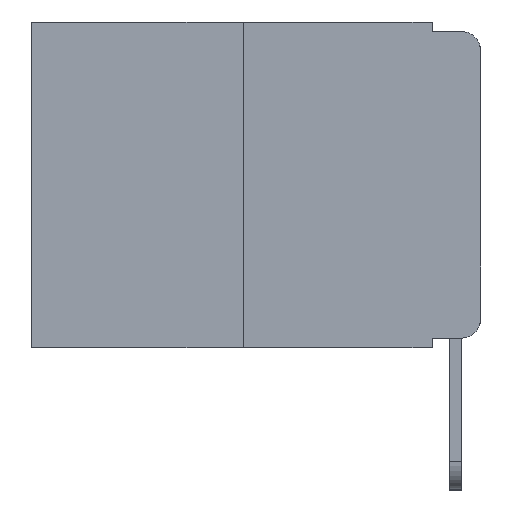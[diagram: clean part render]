
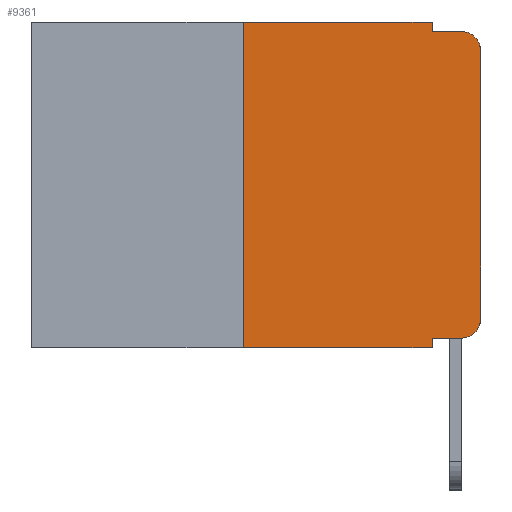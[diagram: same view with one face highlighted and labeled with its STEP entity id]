
A CAD part, left-side view. The second image highlights one B-rep face of the part: STEP entity #9361.
In plain terms, the highlighted planar face has unit normal (-1, 0, 0).
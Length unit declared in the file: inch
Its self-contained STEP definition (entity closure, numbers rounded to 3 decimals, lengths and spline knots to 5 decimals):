
#480 = LINE ( 'NONE', #10778, #15627 ) ;
#1045 = CARTESIAN_POINT ( 'NONE',  ( 0., 0.051, 0. ) ) ;
#1792 = CARTESIAN_POINT ( 'NONE',  ( 0., 0.051, -0.01 ) ) ;
#1855 = DIRECTION ( 'NONE',  ( 0., 0., -1. ) ) ;
#2043 = EDGE_CURVE ( 'NONE', #19481, #11397, #15780, .T. ) ;
#2341 = LINE ( 'NONE', #15578, #12651 ) ;
#2442 = LINE ( 'NONE', #15552, #7257 ) ;
#3213 = DIRECTION ( 'NONE',  ( 0., 0., -1. ) ) ;
#3222 = CARTESIAN_POINT ( 'NONE',  ( 0., 0.02, -0.333 ) ) ;
#4673 = ORIENTED_EDGE ( 'NONE', *, *, #9066, .F. ) ;
#4985 = ORIENTED_EDGE ( 'NONE', *, *, #9174, .F. ) ;
#5011 = ORIENTED_EDGE ( 'NONE', *, *, #9202, .F. ) ;
#5199 = CARTESIAN_POINT ( 'NONE',  ( 0., 0.25, 0. ) ) ;
#5466 = ORIENTED_EDGE ( 'NONE', *, *, #7893, .F. ) ;
#5467 = ORIENTED_EDGE ( 'NONE', *, *, #9296, .T. ) ;
#5751 = VERTEX_POINT ( 'NONE', #23654 ) ;
#5756 = CARTESIAN_POINT ( 'NONE',  ( 0., 0.02, -0.01 ) ) ;
#6042 = VERTEX_POINT ( 'NONE', #3222 ) ;
#6256 = DIRECTION ( 'NONE',  ( 0., 0., 1. ) ) ;
#6399 = ORIENTED_EDGE ( 'NONE', *, *, #9549, .T. ) ;
#6518 = CARTESIAN_POINT ( 'NONE',  ( 0., 0.051, -0.343 ) ) ;
#6658 = AXIS2_PLACEMENT_3D ( 'NONE', #19678, #8766, #21361 ) ;
#6812 = EDGE_CURVE ( 'NONE', #6042, #5751, #7649, .T. ) ;
#6962 = CARTESIAN_POINT ( 'NONE',  ( 0., 0.25, 0. ) ) ;
#7003 = EDGE_CURVE ( 'NONE', #19045, #6042, #480, .T. ) ;
#7114 = CARTESIAN_POINT ( 'NONE',  ( 0., 0.25, -0.343 ) ) ;
#7257 = VECTOR ( 'NONE', #1855, 39.37008 ) ;
#7326 = DIRECTION ( 'NONE',  ( 0., -1., 0. ) ) ;
#7649 = CIRCLE ( 'NONE', #11086, 0.02 ) ;
#7893 = EDGE_CURVE ( 'NONE', #19045, #11397, #2442, .T. ) ;
#8121 = VECTOR ( 'NONE', #3213, 39.37008 ) ;
#8412 = LINE ( 'NONE', #1792, #22184 ) ;
#8766 = DIRECTION ( 'NONE',  ( -1., 0., 0. ) ) ;
#9027 = EDGE_CURVE ( 'NONE', #19481, #18231, #9363, .T. ) ;
#9059 = CIRCLE ( 'NONE', #6658, 0.02 ) ;
#9066 = EDGE_CURVE ( 'NONE', #23045, #13034, #18016, .T. ) ;
#9174 = EDGE_CURVE ( 'NONE', #13034, #21559, #8412, .T. ) ;
#9202 = EDGE_CURVE ( 'NONE', #18231, #23045, #2341, .T. ) ;
#9242 = ORIENTED_EDGE ( 'NONE', *, *, #2043, .T. ) ;
#9296 = EDGE_CURVE ( 'NONE', #11720, #21559, #9059, .T. ) ;
#9361 = ADVANCED_FACE ( 'NONE', ( #20659 ), #16520, .F. ) ;
#9363 = LINE ( 'NONE', #5199, #19080 ) ;
#9549 = EDGE_CURVE ( 'NONE', #5751, #11720, #17179, .T. ) ;
#9937 = DIRECTION ( 'NONE',  ( 0., -1., 0. ) ) ;
#10778 = CARTESIAN_POINT ( 'NONE',  ( 0., 0.051, -0.333 ) ) ;
#10800 = ORIENTED_EDGE ( 'NONE', *, *, #9027, .F. ) ;
#10909 = DIRECTION ( 'NONE',  ( -1., 0., 0. ) ) ;
#11005 = DIRECTION ( 'NONE',  ( 1., 0., 0. ) ) ;
#11086 = AXIS2_PLACEMENT_3D ( 'NONE', #21469, #10909, #23155 ) ;
#11294 = CARTESIAN_POINT ( 'NONE',  ( 0., 0.473, -0.343 ) ) ;
#11397 = VERTEX_POINT ( 'NONE', #6518 ) ;
#11720 = VERTEX_POINT ( 'NONE', #20359 ) ;
#12115 = CARTESIAN_POINT ( 'NONE',  ( 0., 0., 0. ) ) ;
#12622 = DIRECTION ( 'NONE',  ( 0., -1., 0. ) ) ;
#12651 = VECTOR ( 'NONE', #22462, 39.37008 ) ;
#13034 = VERTEX_POINT ( 'NONE', #18909 ) ;
#13080 = ORIENTED_EDGE ( 'NONE', *, *, #7003, .T. ) ;
#14644 = CARTESIAN_POINT ( 'NONE',  ( 0., 0.473, 0. ) ) ;
#15423 = ORIENTED_EDGE ( 'NONE', *, *, #6812, .T. ) ;
#15552 = CARTESIAN_POINT ( 'NONE',  ( 0., 0.051, 0. ) ) ;
#15578 = CARTESIAN_POINT ( 'NONE',  ( 0., 0.473, 0. ) ) ;
#15627 = VECTOR ( 'NONE', #12622, 39.37008 ) ;
#15780 = LINE ( 'NONE', #11294, #19335 ) ;
#16520 = PLANE ( 'NONE',  #19133 ) ;
#16623 = VECTOR ( 'NONE', #6256, 39.37008 ) ;
#17179 = LINE ( 'NONE', #12115, #16623 ) ;
#17546 = CARTESIAN_POINT ( 'NONE',  ( 0., 0.051, -0.333 ) ) ;
#18016 = LINE ( 'NONE', #1045, #8121 ) ;
#18231 = VERTEX_POINT ( 'NONE', #6962 ) ;
#18289 = DIRECTION ( 'NONE',  ( 0., 0., -1. ) ) ;
#18391 = DIRECTION ( 'NONE',  ( 0., 0., 1. ) ) ;
#18619 = EDGE_LOOP ( 'NONE', ( #6399, #5467, #4985, #4673, #5011, #10800, #9242, #5466, #13080, #15423 ) ) ;
#18909 = CARTESIAN_POINT ( 'NONE',  ( 0., 0.051, -0.01 ) ) ;
#19045 = VERTEX_POINT ( 'NONE', #17546 ) ;
#19080 = VECTOR ( 'NONE', #18391, 39.37008 ) ;
#19133 = AXIS2_PLACEMENT_3D ( 'NONE', #14644, #11005, #18289 ) ;
#19335 = VECTOR ( 'NONE', #7326, 39.37008 ) ;
#19400 = CARTESIAN_POINT ( 'NONE',  ( 0., 0.051, 0. ) ) ;
#19481 = VERTEX_POINT ( 'NONE', #7114 ) ;
#19678 = CARTESIAN_POINT ( 'NONE',  ( 0., 0.02, -0.03 ) ) ;
#20359 = CARTESIAN_POINT ( 'NONE',  ( 0., 0., -0.03 ) ) ;
#20659 = FACE_OUTER_BOUND ( 'NONE', #18619, .T. ) ;
#21361 = DIRECTION ( 'NONE',  ( 0., 0., -1. ) ) ;
#21469 = CARTESIAN_POINT ( 'NONE',  ( 0., 0.02, -0.313 ) ) ;
#21559 = VERTEX_POINT ( 'NONE', #5756 ) ;
#22184 = VECTOR ( 'NONE', #9937, 39.37008 ) ;
#22462 = DIRECTION ( 'NONE',  ( 0., -1., 0. ) ) ;
#23045 = VERTEX_POINT ( 'NONE', #19400 ) ;
#23155 = DIRECTION ( 'NONE',  ( 0., 0., -1. ) ) ;
#23654 = CARTESIAN_POINT ( 'NONE',  ( 0., 0., -0.313 ) ) ;
